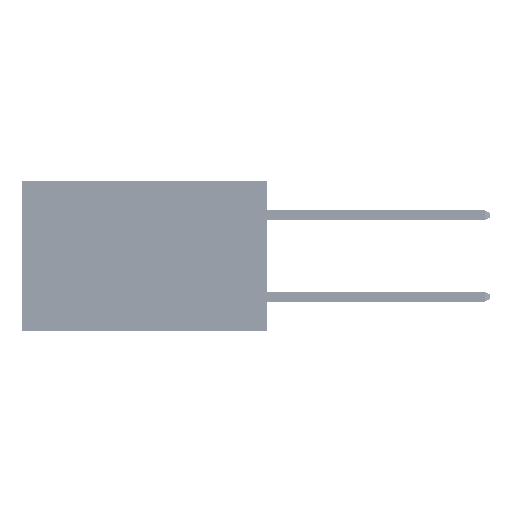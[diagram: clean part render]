
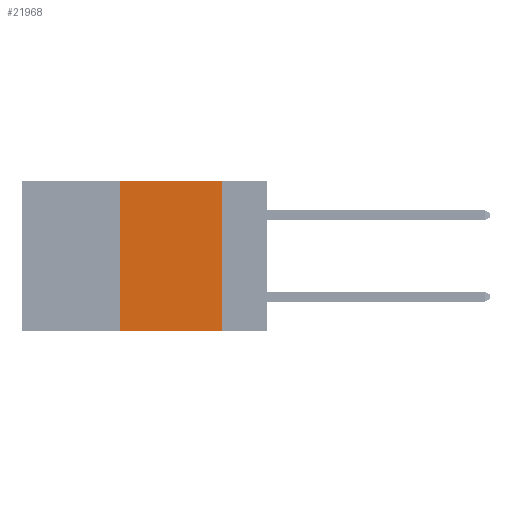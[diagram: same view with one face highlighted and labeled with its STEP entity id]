
A CAD part, left-side view. The second image highlights one B-rep face of the part: STEP entity #21968.
In plain terms, the highlighted planar face has unit normal (-1, 0, 0).
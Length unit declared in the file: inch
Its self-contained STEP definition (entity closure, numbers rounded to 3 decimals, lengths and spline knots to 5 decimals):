
#1716 = DIRECTION ( 'NONE',  ( 0., -1., 0. ) ) ;
#7074 = EDGE_CURVE ( 'NONE', #48478, #25245, #17508, .T. ) ;
#7097 = VERTEX_POINT ( 'NONE', #7742 ) ;
#7485 = VECTOR ( 'NONE', #30113, 39.37008 ) ;
#7742 = CARTESIAN_POINT ( 'NONE',  ( 0., 0.11, -0.37 ) ) ;
#7779 = CARTESIAN_POINT ( 'NONE',  ( 0., 0.11, 0. ) ) ;
#8138 = ORIENTED_EDGE ( 'NONE', *, *, #7074, .F. ) ;
#9474 = CARTESIAN_POINT ( 'NONE',  ( 0., 0.6, -0.37 ) ) ;
#9891 = CARTESIAN_POINT ( 'NONE',  ( 0., 0.11, 0. ) ) ;
#12902 = EDGE_LOOP ( 'NONE', ( #25492, #28613, #8138, #28632 ) ) ;
#12925 = PLANE ( 'NONE',  #47243 ) ;
#14828 = LINE ( 'NONE', #7779, #32438 ) ;
#15082 = EDGE_CURVE ( 'NONE', #48478, #7097, #29258, .T. ) ;
#16338 = CARTESIAN_POINT ( 'NONE',  ( 0., 0.36, 0. ) ) ;
#17508 = LINE ( 'NONE', #30271, #7485 ) ;
#20034 = DIRECTION ( 'NONE',  ( 0., -1., 0. ) ) ;
#20911 = VERTEX_POINT ( 'NONE', #9891 ) ;
#21148 = EDGE_CURVE ( 'NONE', #25245, #20911, #35581, .T. ) ;
#21968 = ADVANCED_FACE ( 'NONE', ( #48616 ), #12925, .F. ) ;
#25046 = EDGE_CURVE ( 'NONE', #20911, #7097, #14828, .T. ) ;
#25245 = VERTEX_POINT ( 'NONE', #16338 ) ;
#25492 = ORIENTED_EDGE ( 'NONE', *, *, #25046, .F. ) ;
#27206 = DIRECTION ( 'NONE',  ( 0., 0., -1. ) ) ;
#27730 = CARTESIAN_POINT ( 'NONE',  ( 0., 0.6, 0. ) ) ;
#27957 = VECTOR ( 'NONE', #20034, 39.37008 ) ;
#28613 = ORIENTED_EDGE ( 'NONE', *, *, #21148, .F. ) ;
#28632 = ORIENTED_EDGE ( 'NONE', *, *, #15082, .T. ) ;
#29258 = LINE ( 'NONE', #9474, #35140 ) ;
#30113 = DIRECTION ( 'NONE',  ( 0., 0., 1. ) ) ;
#30271 = CARTESIAN_POINT ( 'NONE',  ( 0., 0.36, 0. ) ) ;
#31040 = CARTESIAN_POINT ( 'NONE',  ( 0., 0.6, 0. ) ) ;
#32438 = VECTOR ( 'NONE', #27206, 39.37008 ) ;
#35140 = VECTOR ( 'NONE', #1716, 39.37008 ) ;
#35581 = LINE ( 'NONE', #31040, #27957 ) ;
#38891 = DIRECTION ( 'NONE',  ( 0., 0., -1. ) ) ;
#42708 = DIRECTION ( 'NONE',  ( 1., 0., 0. ) ) ;
#44114 = CARTESIAN_POINT ( 'NONE',  ( 0., 0.36, -0.37 ) ) ;
#47243 = AXIS2_PLACEMENT_3D ( 'NONE', #27730, #42708, #38891 ) ;
#48478 = VERTEX_POINT ( 'NONE', #44114 ) ;
#48616 = FACE_OUTER_BOUND ( 'NONE', #12902, .T. ) ;
